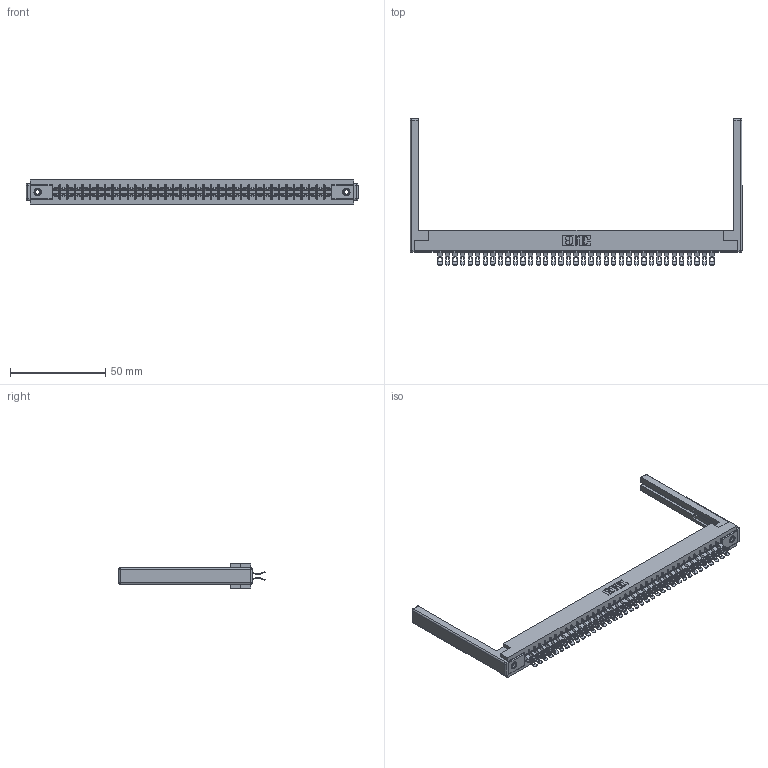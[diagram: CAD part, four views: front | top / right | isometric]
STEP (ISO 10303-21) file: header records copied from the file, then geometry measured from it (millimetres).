
FILE_DESCRIPTION (( 'STEP AP203' ), '1' );
FILE_NAME ('315-074-555-268.STEP', '2019-09-10T22:13:59', ( '' ), ( '' ), 'SwSTEP 2.0', 'SolidWorks 2016', '' );
FILE_SCHEMA (( 'CONFIG_CONTROL_DESIGN' ));
Length unit declared in the file: inch
Products named in the file (5): 307-220-068; 315-074-555-268; 345-250-001_345-250-001-102; 305 Part_.156 Dia; 305-290-001_555
Assembly tree (79 placements, depth 2):
  315-074-555-268
    305 Part_.156 Dia
    305-290-001_555  x74
    345-250-001_345-250-001-102  x2
    307-220-068  x2
Bounding box: 174.04 x 76.71 x 12.7 mm (x, y, z)
Volume: 22736.9 mm3; surface area: 28585.8 mm2
Topology: 79 solids, 79 shells, 5154 faces, 15321 edges, 9994 vertices
Faces by surface type: plane 2524, cylinder 2458, sphere 156, cone 12, torus 4
Entity records: 44053 total; most frequent: CARTESIAN_POINT 7280, ORIENTED_EDGE 7208, DIRECTION 7060, EDGE_CURVE 3604, VECTOR 2880, LINE 2880, VERTEX_POINT 2294, AXIS2_PLACEMENT_3D 2090
